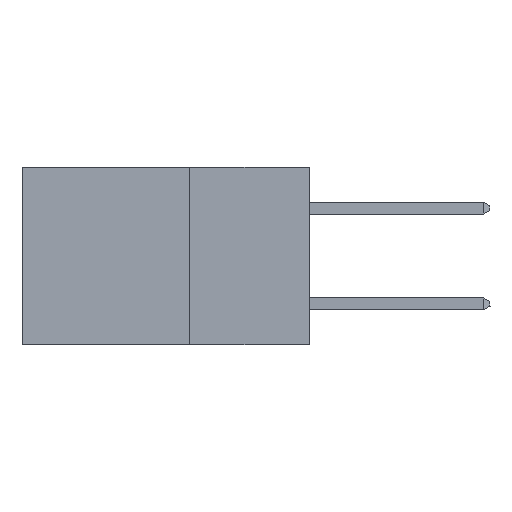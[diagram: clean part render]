
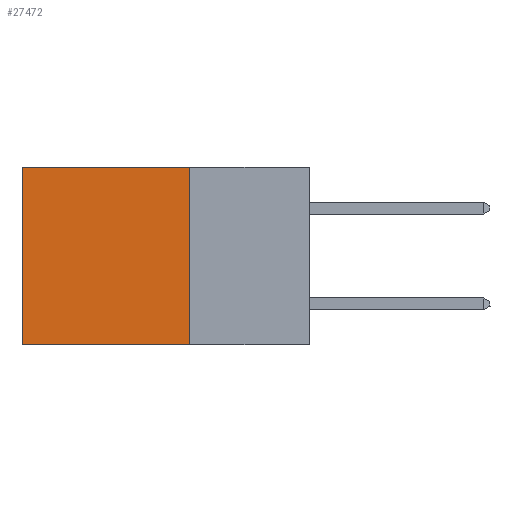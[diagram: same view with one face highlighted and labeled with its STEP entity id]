
A CAD part, left-side view. The second image highlights one B-rep face of the part: STEP entity #27472.
In plain terms, the highlighted planar face has unit normal (-1, 0, 0).
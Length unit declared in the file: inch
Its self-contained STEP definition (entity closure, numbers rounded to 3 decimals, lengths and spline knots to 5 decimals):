
#466 = ORIENTED_EDGE ( 'NONE', *, *, #10421, .F. ) ;
#1948 = EDGE_CURVE ( 'NONE', #28631, #5677, #9294, .T. ) ;
#2320 = CARTESIAN_POINT ( 'NONE',  ( 0.2875, 0.25, 0. ) ) ;
#3513 = CARTESIAN_POINT ( 'NONE',  ( 0.2875, 0.25, 0. ) ) ;
#3600 = VECTOR ( 'NONE', #5394, 39.37008 ) ;
#5394 = DIRECTION ( 'NONE',  ( 0., 0., -1. ) ) ;
#5420 = EDGE_LOOP ( 'NONE', ( #7688, #28980, #466, #12434 ) ) ;
#5677 = VERTEX_POINT ( 'NONE', #6235 ) ;
#5878 = LINE ( 'NONE', #30759, #18994 ) ;
#6235 = CARTESIAN_POINT ( 'NONE',  ( 0.2875, 0.6, -0.37 ) ) ;
#6958 = AXIS2_PLACEMENT_3D ( 'NONE', #3513, #22589, #8116 ) ;
#7688 = ORIENTED_EDGE ( 'NONE', *, *, #10173, .T. ) ;
#8116 = DIRECTION ( 'NONE',  ( 0., 0., -1. ) ) ;
#9294 = LINE ( 'NONE', #28875, #15708 ) ;
#10173 = EDGE_CURVE ( 'NONE', #14995, #5677, #26846, .T. ) ;
#10324 = DIRECTION ( 'NONE',  ( 0., 1., 0. ) ) ;
#10421 = EDGE_CURVE ( 'NONE', #13907, #28631, #22344, .T. ) ;
#11528 = CARTESIAN_POINT ( 'NONE',  ( 0.2875, 0.6, 0. ) ) ;
#12434 = ORIENTED_EDGE ( 'NONE', *, *, #12529, .T. ) ;
#12529 = EDGE_CURVE ( 'NONE', #13907, #14995, #5878, .T. ) ;
#13185 = PLANE ( 'NONE',  #6958 ) ;
#13907 = VERTEX_POINT ( 'NONE', #25151 ) ;
#14995 = VERTEX_POINT ( 'NONE', #11528 ) ;
#15708 = VECTOR ( 'NONE', #19337, 39.37008 ) ;
#15983 = VECTOR ( 'NONE', #28758, 39.37008 ) ;
#18994 = VECTOR ( 'NONE', #10324, 39.37008 ) ;
#19337 = DIRECTION ( 'NONE',  ( 0., 1., 0. ) ) ;
#19660 = CARTESIAN_POINT ( 'NONE',  ( 0.2875, 0.6, 0. ) ) ;
#20046 = FACE_OUTER_BOUND ( 'NONE', #5420, .T. ) ;
#21472 = CARTESIAN_POINT ( 'NONE',  ( 0.2875, 0.25, -0.37 ) ) ;
#22344 = LINE ( 'NONE', #2320, #15983 ) ;
#22589 = DIRECTION ( 'NONE',  ( 1., 0., 0. ) ) ;
#25151 = CARTESIAN_POINT ( 'NONE',  ( 0.2875, 0.25, 0. ) ) ;
#26846 = LINE ( 'NONE', #19660, #3600 ) ;
#27472 = ADVANCED_FACE ( 'NONE', ( #20046 ), #13185, .F. ) ;
#28631 = VERTEX_POINT ( 'NONE', #21472 ) ;
#28758 = DIRECTION ( 'NONE',  ( 0., 0., -1. ) ) ;
#28875 = CARTESIAN_POINT ( 'NONE',  ( 0.2875, 0.25, -0.37 ) ) ;
#28980 = ORIENTED_EDGE ( 'NONE', *, *, #1948, .F. ) ;
#30759 = CARTESIAN_POINT ( 'NONE',  ( 0.2875, 0.25, 0. ) ) ;
